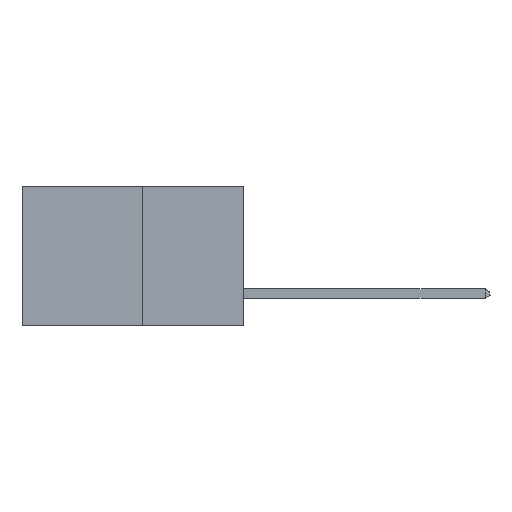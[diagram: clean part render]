
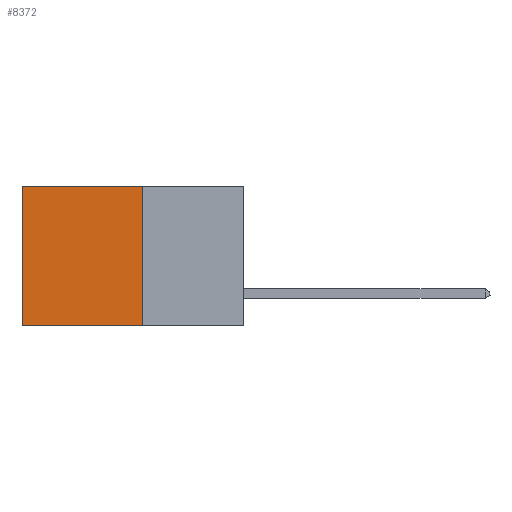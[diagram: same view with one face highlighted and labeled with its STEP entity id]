
A CAD part, left-side view. The second image highlights one B-rep face of the part: STEP entity #8372.
In plain terms, the highlighted planar face has unit normal (-1, 0, 0).
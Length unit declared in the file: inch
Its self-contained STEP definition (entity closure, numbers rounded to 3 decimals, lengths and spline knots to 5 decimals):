
#216 = EDGE_CURVE ( 'NONE', #8356, #518, #16002, .T. ) ;
#518 = VERTEX_POINT ( 'NONE', #16579 ) ;
#1664 = VECTOR ( 'NONE', #12663, 39.37008 ) ;
#4782 = CARTESIAN_POINT ( 'NONE',  ( 0.277, 0.27, -0.37 ) ) ;
#4827 = VERTEX_POINT ( 'NONE', #13777 ) ;
#4973 = PLANE ( 'NONE',  #5015 ) ;
#5015 = AXIS2_PLACEMENT_3D ( 'NONE', #12590, #6894, #20257 ) ;
#6445 = VECTOR ( 'NONE', #10034, 39.37008 ) ;
#6692 = FACE_OUTER_BOUND ( 'NONE', #20206, .T. ) ;
#6894 = DIRECTION ( 'NONE',  ( 1., 0., 0. ) ) ;
#8356 = VERTEX_POINT ( 'NONE', #23997 ) ;
#8372 = ADVANCED_FACE ( 'NONE', ( #6692 ), #4973, .F. ) ;
#8375 = ORIENTED_EDGE ( 'NONE', *, *, #17602, .F. ) ;
#8540 = DIRECTION ( 'NONE',  ( 0., 1., 0. ) ) ;
#10034 = DIRECTION ( 'NONE',  ( 0., 0., -1. ) ) ;
#10068 = CARTESIAN_POINT ( 'NONE',  ( 0.277, 0.59, -0.37 ) ) ;
#11050 = VECTOR ( 'NONE', #8540, 39.37008 ) ;
#11261 = LINE ( 'NONE', #14513, #1664 ) ;
#12215 = CARTESIAN_POINT ( 'NONE',  ( 0.277, 0.27, -0.37 ) ) ;
#12522 = VERTEX_POINT ( 'NONE', #4782 ) ;
#12590 = CARTESIAN_POINT ( 'NONE',  ( 0.277, 0.27, -0.37 ) ) ;
#12663 = DIRECTION ( 'NONE',  ( 0., 1., 0. ) ) ;
#12984 = VECTOR ( 'NONE', #23641, 39.37008 ) ;
#13577 = EDGE_CURVE ( 'NONE', #12522, #518, #11261, .T. ) ;
#13777 = CARTESIAN_POINT ( 'NONE',  ( 0.277, 0.27, 0. ) ) ;
#14513 = CARTESIAN_POINT ( 'NONE',  ( 0.277, 0.27, -0.37 ) ) ;
#15372 = ORIENTED_EDGE ( 'NONE', *, *, #20074, .T. ) ;
#15886 = ORIENTED_EDGE ( 'NONE', *, *, #216, .T. ) ;
#16002 = LINE ( 'NONE', #10068, #6445 ) ;
#16105 = LINE ( 'NONE', #18033, #11050 ) ;
#16579 = CARTESIAN_POINT ( 'NONE',  ( 0.277, 0.59, -0.37 ) ) ;
#17602 = EDGE_CURVE ( 'NONE', #4827, #12522, #18653, .T. ) ;
#18033 = CARTESIAN_POINT ( 'NONE',  ( 0.277, 0.27, 0. ) ) ;
#18653 = LINE ( 'NONE', #12215, #12984 ) ;
#20074 = EDGE_CURVE ( 'NONE', #4827, #8356, #16105, .T. ) ;
#20206 = EDGE_LOOP ( 'NONE', ( #15886, #24357, #8375, #15372 ) ) ;
#20257 = DIRECTION ( 'NONE',  ( 0., 0., -1. ) ) ;
#23641 = DIRECTION ( 'NONE',  ( 0., 0., -1. ) ) ;
#23997 = CARTESIAN_POINT ( 'NONE',  ( 0.277, 0.59, 0. ) ) ;
#24357 = ORIENTED_EDGE ( 'NONE', *, *, #13577, .F. ) ;
